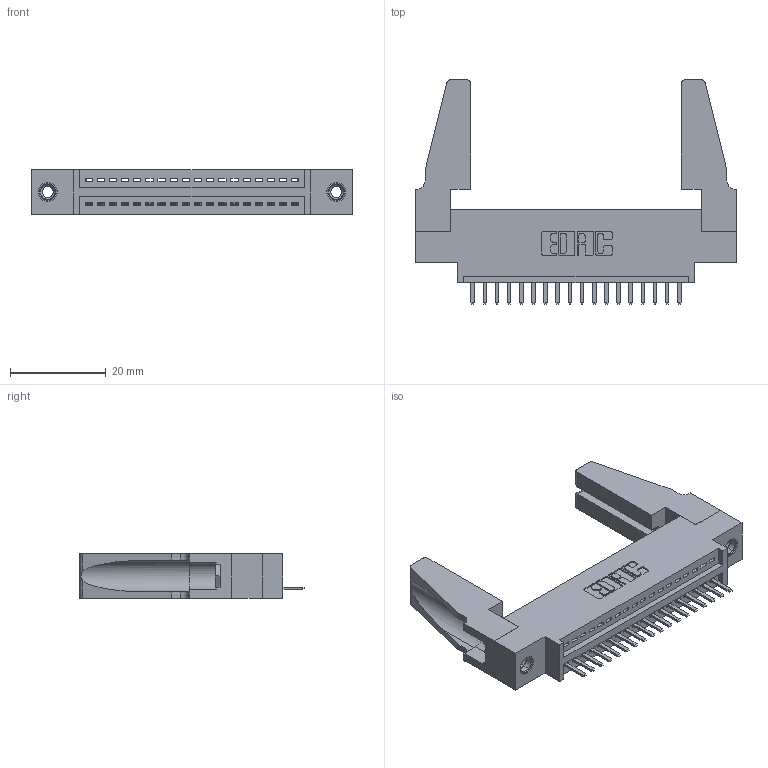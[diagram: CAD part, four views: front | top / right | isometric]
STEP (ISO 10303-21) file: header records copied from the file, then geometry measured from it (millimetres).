
FILE_DESCRIPTION (( 'STEP AP203' ), '1' );
FILE_NAME ('395-018-520-688.STEP', '2019-10-17T15:18:33', ( '' ), ( '' ), 'SwSTEP 2.0', 'SolidWorks 2016', '' );
FILE_SCHEMA (( 'CONFIG_CONTROL_DESIGN' ));
Length unit declared in the file: inch
Products named in the file (5): 395-018-520-688; 345 Part_0.170 Offset - 0.156 Dia-TH; 345-292-001_345-293-120; 345-250-001_345-250-001-102; 345-220-078_345-220-088
Assembly tree (23 placements, depth 2):
  395-018-520-688
    345 Part_0.170 Offset - 0.156 Dia-TH
    345-292-001_345-293-120  x18
    345-250-001_345-250-001-102  x2
    345-220-078_345-220-088  x2
Bounding box: 66.95 x 46.86 x 9.4 mm (x, y, z)
Volume: 9250.1 mm3; surface area: 10730.6 mm2
Topology: 23 solids, 23 shells, 1370 faces, 3979 edges, 2594 vertices
Faces by surface type: plane 912, cylinder 442, cone 12, torus 4
Entity records: 19172 total; most frequent: CARTESIAN_POINT 3324, ORIENTED_EDGE 3224, DIRECTION 2932, EDGE_CURVE 1612, LINE 1362, VECTOR 1362, VERTEX_POINT 1066, AXIS2_PLACEMENT_3D 785
